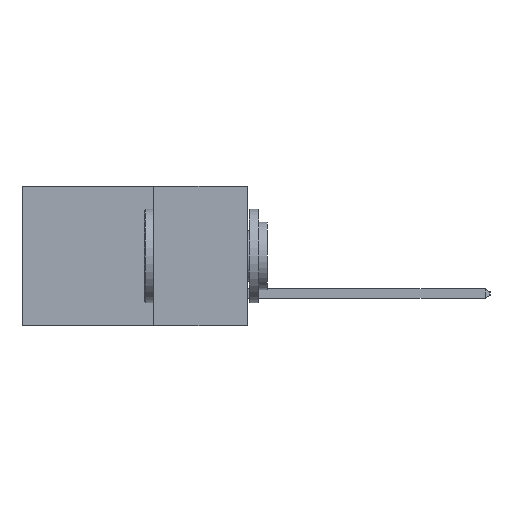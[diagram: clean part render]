
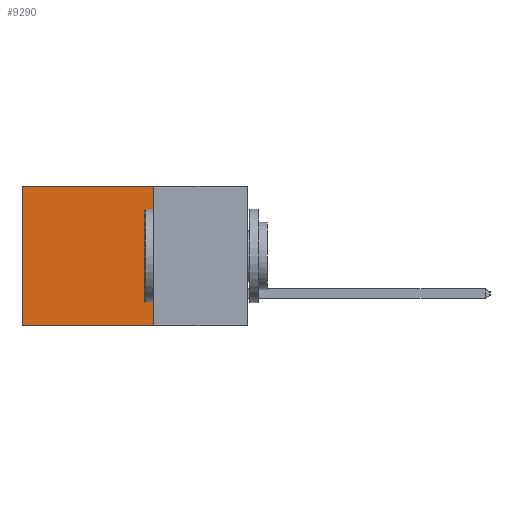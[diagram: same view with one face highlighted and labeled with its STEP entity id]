
A CAD part, left-side view. The second image highlights one B-rep face of the part: STEP entity #9290.
In plain terms, the highlighted planar face has unit normal (-1, 0, 0).
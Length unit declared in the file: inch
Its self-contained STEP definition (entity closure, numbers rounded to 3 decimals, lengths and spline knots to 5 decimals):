
#100 = EDGE_LOOP ( 'NONE', ( #9121, #6310, #9194, #9754 ) ) ;
#178 = DIRECTION ( 'NONE',  ( 0., 1., 0. ) ) ;
#290 = VECTOR ( 'NONE', #9447, 39.37008 ) ;
#311 = CARTESIAN_POINT ( 'NONE',  ( 0.298, 0.25, 0. ) ) ;
#325 = CARTESIAN_POINT ( 'NONE',  ( 0.298, 0.25, 0. ) ) ;
#952 = DIRECTION ( 'NONE',  ( 1., 0., 0. ) ) ;
#1401 = VERTEX_POINT ( 'NONE', #9565 ) ;
#1631 = LINE ( 'NONE', #4556, #10861 ) ;
#2629 = VERTEX_POINT ( 'NONE', #9577 ) ;
#3148 = EDGE_CURVE ( 'NONE', #1401, #6842, #7848, .T. ) ;
#3211 = FACE_OUTER_BOUND ( 'NONE', #100, .T. ) ;
#3610 = VERTEX_POINT ( 'NONE', #9182 ) ;
#3826 = CARTESIAN_POINT ( 'NONE',  ( 0.298, 0.6, -0.37 ) ) ;
#4556 = CARTESIAN_POINT ( 'NONE',  ( 0.298, 0.6, 0. ) ) ;
#5003 = DIRECTION ( 'NONE',  ( 0., 0., -1. ) ) ;
#5017 = EDGE_CURVE ( 'NONE', #2629, #6842, #1631, .T. ) ;
#6310 = ORIENTED_EDGE ( 'NONE', *, *, #3148, .F. ) ;
#6842 = VERTEX_POINT ( 'NONE', #3826 ) ;
#7023 = EDGE_CURVE ( 'NONE', #3610, #1401, #9840, .T. ) ;
#7441 = DIRECTION ( 'NONE',  ( 0., 0., -1. ) ) ;
#7578 = VECTOR ( 'NONE', #5003, 39.37008 ) ;
#7716 = EDGE_CURVE ( 'NONE', #3610, #2629, #9971, .T. ) ;
#7848 = LINE ( 'NONE', #10912, #9567 ) ;
#7869 = DIRECTION ( 'NONE',  ( 0., 0., -1. ) ) ;
#8986 = AXIS2_PLACEMENT_3D ( 'NONE', #9115, #952, #7441 ) ;
#9115 = CARTESIAN_POINT ( 'NONE',  ( 0.298, 0.25, 0. ) ) ;
#9121 = ORIENTED_EDGE ( 'NONE', *, *, #5017, .T. ) ;
#9182 = CARTESIAN_POINT ( 'NONE',  ( 0.298, 0.25, 0. ) ) ;
#9194 = ORIENTED_EDGE ( 'NONE', *, *, #7023, .F. ) ;
#9290 = ADVANCED_FACE ( 'NONE', ( #3211 ), #11646, .F. ) ;
#9447 = DIRECTION ( 'NONE',  ( 0., 1., 0. ) ) ;
#9565 = CARTESIAN_POINT ( 'NONE',  ( 0.298, 0.25, -0.37 ) ) ;
#9567 = VECTOR ( 'NONE', #178, 39.37008 ) ;
#9577 = CARTESIAN_POINT ( 'NONE',  ( 0.298, 0.6, 0. ) ) ;
#9754 = ORIENTED_EDGE ( 'NONE', *, *, #7716, .T. ) ;
#9840 = LINE ( 'NONE', #325, #7578 ) ;
#9971 = LINE ( 'NONE', #311, #290 ) ;
#10861 = VECTOR ( 'NONE', #7869, 39.37008 ) ;
#10912 = CARTESIAN_POINT ( 'NONE',  ( 0.298, 0.25, -0.37 ) ) ;
#11646 = PLANE ( 'NONE',  #8986 ) ;
